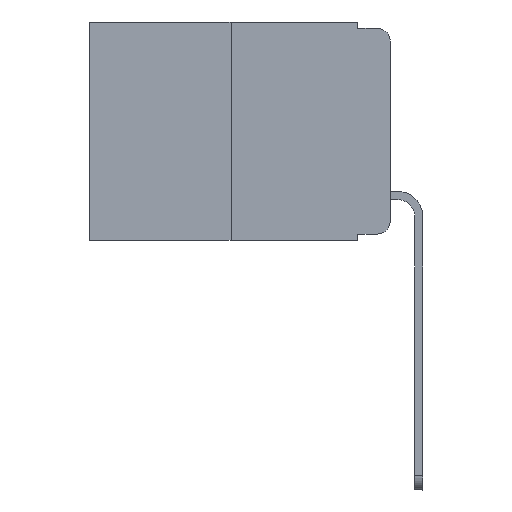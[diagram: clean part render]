
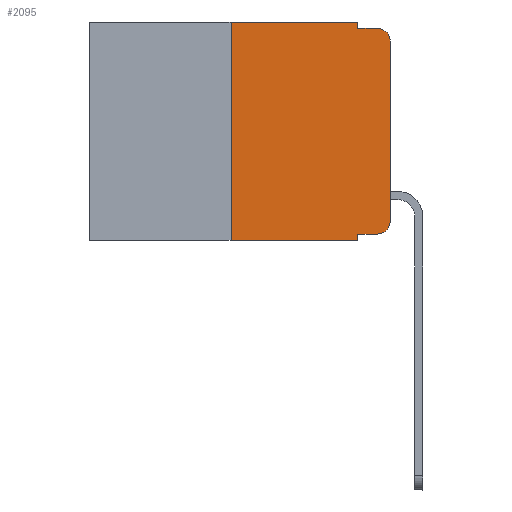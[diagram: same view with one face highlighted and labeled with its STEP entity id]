
A CAD part, left-side view. The second image highlights one B-rep face of the part: STEP entity #2095.
In plain terms, the highlighted planar face has unit normal (-1, 0, 0).
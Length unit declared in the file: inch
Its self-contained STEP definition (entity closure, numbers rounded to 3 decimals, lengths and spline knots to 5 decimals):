
#32 = EDGE_CURVE ( 'NONE', #9034, #2224, #475, .T. ) ;
#111 = LINE ( 'NONE', #1910, #10168 ) ;
#229 = DIRECTION ( 'NONE',  ( 0., 0., -1. ) ) ;
#322 = AXIS2_PLACEMENT_3D ( 'NONE', #4322, #7582, #4144 ) ;
#475 = LINE ( 'NONE', #5588, #9961 ) ;
#930 = VERTEX_POINT ( 'NONE', #7474 ) ;
#996 = DIRECTION ( 'NONE',  ( -1., 0., 0. ) ) ;
#1160 = LINE ( 'NONE', #8236, #6510 ) ;
#1389 = CARTESIAN_POINT ( 'NONE',  ( 0., 0.051, -0.343 ) ) ;
#1576 = VERTEX_POINT ( 'NONE', #7272 ) ;
#1839 = CARTESIAN_POINT ( 'NONE',  ( 0., 0.051, 0. ) ) ;
#1851 = CARTESIAN_POINT ( 'NONE',  ( 0., 0.02, -0.313 ) ) ;
#1910 = CARTESIAN_POINT ( 'NONE',  ( 0., 0.051, -0.01 ) ) ;
#1935 = ORIENTED_EDGE ( 'NONE', *, *, #5395, .T. ) ;
#2095 = ADVANCED_FACE ( 'NONE', ( #5851 ), #10288, .F. ) ;
#2098 = EDGE_CURVE ( 'NONE', #1576, #10210, #2552, .T. ) ;
#2135 = DIRECTION ( 'NONE',  ( 0., 0., 1. ) ) ;
#2224 = VERTEX_POINT ( 'NONE', #3563 ) ;
#2360 = EDGE_CURVE ( 'NONE', #2224, #930, #1160, .T. ) ;
#2364 = AXIS2_PLACEMENT_3D ( 'NONE', #1851, #996, #4536 ) ;
#2552 = LINE ( 'NONE', #9326, #5058 ) ;
#2922 = EDGE_CURVE ( 'NONE', #10210, #11171, #10981, .T. ) ;
#3080 = LINE ( 'NONE', #9908, #5610 ) ;
#3374 = ORIENTED_EDGE ( 'NONE', *, *, #2922, .T. ) ;
#3563 = CARTESIAN_POINT ( 'NONE',  ( 0., 0.25, 0. ) ) ;
#3774 = ORIENTED_EDGE ( 'NONE', *, *, #4439, .T. ) ;
#4045 = VECTOR ( 'NONE', #229, 39.37008 ) ;
#4144 = DIRECTION ( 'NONE',  ( 0., 0., -1. ) ) ;
#4283 = DIRECTION ( 'NONE',  ( 0., -1., 0. ) ) ;
#4302 = DIRECTION ( 'NONE',  ( 0., 0., -1. ) ) ;
#4322 = CARTESIAN_POINT ( 'NONE',  ( 0., 0.473, 0. ) ) ;
#4423 = DIRECTION ( 'NONE',  ( 0., 0., -1. ) ) ;
#4439 = EDGE_CURVE ( 'NONE', #9369, #8347, #3080, .T. ) ;
#4529 = ORIENTED_EDGE ( 'NONE', *, *, #5426, .F. ) ;
#4536 = DIRECTION ( 'NONE',  ( 0., 0., -1. ) ) ;
#4550 = CARTESIAN_POINT ( 'NONE',  ( 0., 0.473, -0.343 ) ) ;
#4570 = VECTOR ( 'NONE', #8074, 39.37008 ) ;
#5058 = VECTOR ( 'NONE', #5107, 39.37008 ) ;
#5107 = DIRECTION ( 'NONE',  ( 0., 0., 1. ) ) ;
#5218 = ORIENTED_EDGE ( 'NONE', *, *, #2098, .T. ) ;
#5276 = CARTESIAN_POINT ( 'NONE',  ( 0., 0.02, -0.01 ) ) ;
#5391 = AXIS2_PLACEMENT_3D ( 'NONE', #9181, #10211, #4302 ) ;
#5395 = EDGE_CURVE ( 'NONE', #8347, #1576, #6713, .T. ) ;
#5426 = EDGE_CURVE ( 'NONE', #930, #9989, #7793, .T. ) ;
#5451 = CARTESIAN_POINT ( 'NONE',  ( 0., 0.051, 0. ) ) ;
#5587 = ORIENTED_EDGE ( 'NONE', *, *, #8813, .F. ) ;
#5588 = CARTESIAN_POINT ( 'NONE',  ( 0., 0.25, 0. ) ) ;
#5610 = VECTOR ( 'NONE', #9734, 39.37008 ) ;
#5851 = FACE_OUTER_BOUND ( 'NONE', #6016, .T. ) ;
#5988 = VERTEX_POINT ( 'NONE', #1389 ) ;
#6016 = EDGE_LOOP ( 'NONE', ( #5218, #3374, #5587, #4529, #10158, #8315, #6350, #6553, #3774, #1935 ) ) ;
#6172 = VECTOR ( 'NONE', #4423, 39.37008 ) ;
#6350 = ORIENTED_EDGE ( 'NONE', *, *, #7758, .T. ) ;
#6405 = CARTESIAN_POINT ( 'NONE',  ( 0., 0.25, -0.343 ) ) ;
#6449 = DIRECTION ( 'NONE',  ( 0., -1., 0. ) ) ;
#6510 = VECTOR ( 'NONE', #6449, 39.37008 ) ;
#6553 = ORIENTED_EDGE ( 'NONE', *, *, #7305, .F. ) ;
#6713 = CIRCLE ( 'NONE', #2364, 0.02 ) ;
#6788 = CARTESIAN_POINT ( 'NONE',  ( 0., 0., -0.03 ) ) ;
#7272 = CARTESIAN_POINT ( 'NONE',  ( 0., 0., -0.313 ) ) ;
#7305 = EDGE_CURVE ( 'NONE', #9369, #5988, #7987, .T. ) ;
#7474 = CARTESIAN_POINT ( 'NONE',  ( 0., 0.051, 0. ) ) ;
#7582 = DIRECTION ( 'NONE',  ( 1., 0., 0. ) ) ;
#7606 = CARTESIAN_POINT ( 'NONE',  ( 0., 0.02, -0.333 ) ) ;
#7758 = EDGE_CURVE ( 'NONE', #9034, #5988, #10515, .T. ) ;
#7793 = LINE ( 'NONE', #1839, #6172 ) ;
#7987 = LINE ( 'NONE', #5451, #4045 ) ;
#8074 = DIRECTION ( 'NONE',  ( 0., -1., 0. ) ) ;
#8236 = CARTESIAN_POINT ( 'NONE',  ( 0., 0.473, 0. ) ) ;
#8315 = ORIENTED_EDGE ( 'NONE', *, *, #32, .F. ) ;
#8347 = VERTEX_POINT ( 'NONE', #7606 ) ;
#8813 = EDGE_CURVE ( 'NONE', #9989, #11171, #111, .T. ) ;
#9034 = VERTEX_POINT ( 'NONE', #6405 ) ;
#9181 = CARTESIAN_POINT ( 'NONE',  ( 0., 0.02, -0.03 ) ) ;
#9326 = CARTESIAN_POINT ( 'NONE',  ( 0., 0., 0. ) ) ;
#9369 = VERTEX_POINT ( 'NONE', #10105 ) ;
#9734 = DIRECTION ( 'NONE',  ( 0., -1., 0. ) ) ;
#9908 = CARTESIAN_POINT ( 'NONE',  ( 0., 0.051, -0.333 ) ) ;
#9961 = VECTOR ( 'NONE', #2135, 39.37008 ) ;
#9989 = VERTEX_POINT ( 'NONE', #9993 ) ;
#9993 = CARTESIAN_POINT ( 'NONE',  ( 0., 0.051, -0.01 ) ) ;
#10105 = CARTESIAN_POINT ( 'NONE',  ( 0., 0.051, -0.333 ) ) ;
#10158 = ORIENTED_EDGE ( 'NONE', *, *, #2360, .F. ) ;
#10168 = VECTOR ( 'NONE', #4283, 39.37008 ) ;
#10210 = VERTEX_POINT ( 'NONE', #6788 ) ;
#10211 = DIRECTION ( 'NONE',  ( -1., 0., 0. ) ) ;
#10288 = PLANE ( 'NONE',  #322 ) ;
#10515 = LINE ( 'NONE', #4550, #4570 ) ;
#10981 = CIRCLE ( 'NONE', #5391, 0.02 ) ;
#11171 = VERTEX_POINT ( 'NONE', #5276 ) ;
